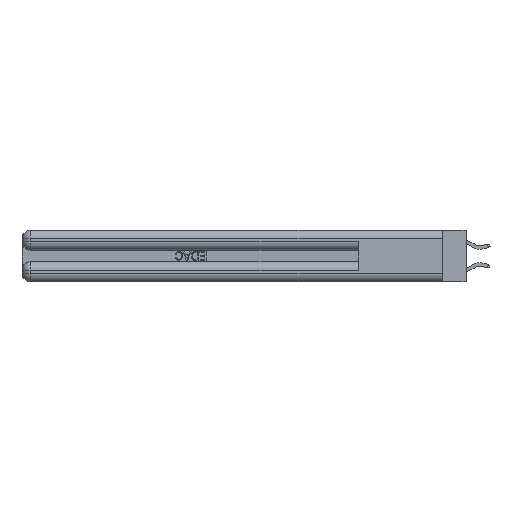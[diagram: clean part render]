
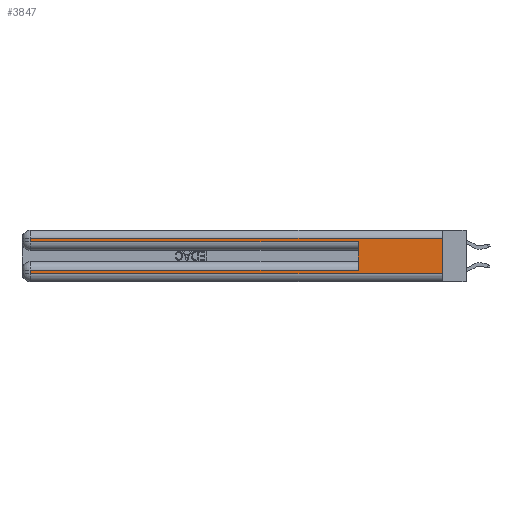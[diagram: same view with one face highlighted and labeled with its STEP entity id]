
A CAD part, left-side view. The second image highlights one B-rep face of the part: STEP entity #3847.
In plain terms, the highlighted planar face has unit normal (-1, 0, 0).
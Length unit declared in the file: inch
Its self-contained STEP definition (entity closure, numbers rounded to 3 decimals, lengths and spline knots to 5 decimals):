
#159 = VERTEX_POINT ( 'NONE', #21411 ) ;
#930 = CARTESIAN_POINT ( 'NONE',  ( 0., 2.94, 0.31 ) ) ;
#2586 = EDGE_CURVE ( 'NONE', #5223, #3981, #11230, .T. ) ;
#2915 = VECTOR ( 'NONE', #15169, 39.37008 ) ;
#3310 = DIRECTION ( 'NONE',  ( 0., 0., -1. ) ) ;
#3345 = EDGE_LOOP ( 'NONE', ( #12066, #18099, #30563, #4574, #16360, #20269, #9818, #15559 ) ) ;
#3847 = ADVANCED_FACE ( 'NONE', ( #15359 ), #16615, .F. ) ;
#3981 = VERTEX_POINT ( 'NONE', #24845 ) ;
#4574 = ORIENTED_EDGE ( 'NONE', *, *, #2586, .T. ) ;
#4626 = DIRECTION ( 'NONE',  ( 0., 0., -1. ) ) ;
#5223 = VERTEX_POINT ( 'NONE', #12116 ) ;
#5605 = EDGE_CURVE ( 'NONE', #159, #30603, #14105, .T. ) ;
#5897 = CARTESIAN_POINT ( 'NONE',  ( 0., 2.94, 0.06 ) ) ;
#6572 = EDGE_CURVE ( 'NONE', #7374, #24422, #9858, .T. ) ;
#6968 = DIRECTION ( 'NONE',  ( 1., 0., 0. ) ) ;
#7374 = VERTEX_POINT ( 'NONE', #14936 ) ;
#8783 = VERTEX_POINT ( 'NONE', #930 ) ;
#9000 = AXIS2_PLACEMENT_3D ( 'NONE', #11763, #6968, #23907 ) ;
#9295 = LINE ( 'NONE', #10842, #21410 ) ;
#9398 = LINE ( 'NONE', #12736, #2915 ) ;
#9818 = ORIENTED_EDGE ( 'NONE', *, *, #22522, .T. ) ;
#9858 = LINE ( 'NONE', #26166, #21970 ) ;
#10017 = DIRECTION ( 'NONE',  ( 0., 1., 0. ) ) ;
#10842 = CARTESIAN_POINT ( 'NONE',  ( 0., 0., 0.06 ) ) ;
#11230 = LINE ( 'NONE', #13934, #29784 ) ;
#11763 = CARTESIAN_POINT ( 'NONE',  ( 0., 0., 0.37 ) ) ;
#12066 = ORIENTED_EDGE ( 'NONE', *, *, #5605, .F. ) ;
#12116 = CARTESIAN_POINT ( 'NONE',  ( 0., 2.94, 0.285 ) ) ;
#12736 = CARTESIAN_POINT ( 'NONE',  ( 0., 0.6, 0.145 ) ) ;
#12997 = CARTESIAN_POINT ( 'NONE',  ( 0., 0., 0.37 ) ) ;
#13303 = EDGE_CURVE ( 'NONE', #8783, #5223, #31023, .T. ) ;
#13833 = DIRECTION ( 'NONE',  ( 0., -1., 0. ) ) ;
#13934 = CARTESIAN_POINT ( 'NONE',  ( 0., 0., 0.285 ) ) ;
#13986 = CARTESIAN_POINT ( 'NONE',  ( 0., 2.94, 0.085 ) ) ;
#14105 = LINE ( 'NONE', #12997, #26977 ) ;
#14798 = CARTESIAN_POINT ( 'NONE',  ( 0., 0., 0.31 ) ) ;
#14936 = CARTESIAN_POINT ( 'NONE',  ( 0., 0.6, 0.085 ) ) ;
#15169 = DIRECTION ( 'NONE',  ( 0., 0., 1. ) ) ;
#15359 = FACE_OUTER_BOUND ( 'NONE', #3345, .T. ) ;
#15382 = EDGE_CURVE ( 'NONE', #16833, #30603, #9295, .T. ) ;
#15559 = ORIENTED_EDGE ( 'NONE', *, *, #15382, .T. ) ;
#16360 = ORIENTED_EDGE ( 'NONE', *, *, #22108, .F. ) ;
#16615 = PLANE ( 'NONE',  #9000 ) ;
#16729 = CARTESIAN_POINT ( 'NONE',  ( 0., 2.94, 0.37 ) ) ;
#16833 = VERTEX_POINT ( 'NONE', #5897 ) ;
#17827 = DIRECTION ( 'NONE',  ( 0., 0., -1. ) ) ;
#18099 = ORIENTED_EDGE ( 'NONE', *, *, #23309, .T. ) ;
#18671 = CARTESIAN_POINT ( 'NONE',  ( 0., 0., 0.06 ) ) ;
#20269 = ORIENTED_EDGE ( 'NONE', *, *, #6572, .T. ) ;
#20307 = VECTOR ( 'NONE', #10017, 39.37008 ) ;
#21061 = LINE ( 'NONE', #14798, #20307 ) ;
#21408 = DIRECTION ( 'NONE',  ( 0., 1., 0. ) ) ;
#21410 = VECTOR ( 'NONE', #27868, 39.37008 ) ;
#21411 = CARTESIAN_POINT ( 'NONE',  ( 0., 0., 0.31 ) ) ;
#21970 = VECTOR ( 'NONE', #21408, 39.37008 ) ;
#22108 = EDGE_CURVE ( 'NONE', #7374, #3981, #9398, .T. ) ;
#22522 = EDGE_CURVE ( 'NONE', #24422, #16833, #23761, .T. ) ;
#23309 = EDGE_CURVE ( 'NONE', #159, #8783, #21061, .T. ) ;
#23761 = LINE ( 'NONE', #16729, #28707 ) ;
#23907 = DIRECTION ( 'NONE',  ( 0., 0., -1. ) ) ;
#24422 = VERTEX_POINT ( 'NONE', #13986 ) ;
#24554 = VECTOR ( 'NONE', #17827, 39.37008 ) ;
#24845 = CARTESIAN_POINT ( 'NONE',  ( 0., 0.6, 0.285 ) ) ;
#26166 = CARTESIAN_POINT ( 'NONE',  ( 0., 0., 0.085 ) ) ;
#26977 = VECTOR ( 'NONE', #3310, 39.37008 ) ;
#27451 = CARTESIAN_POINT ( 'NONE',  ( 0., 2.94, 0.37 ) ) ;
#27868 = DIRECTION ( 'NONE',  ( 0., -1., 0. ) ) ;
#28707 = VECTOR ( 'NONE', #4626, 39.37008 ) ;
#29784 = VECTOR ( 'NONE', #13833, 39.37008 ) ;
#30563 = ORIENTED_EDGE ( 'NONE', *, *, #13303, .T. ) ;
#30603 = VERTEX_POINT ( 'NONE', #18671 ) ;
#31023 = LINE ( 'NONE', #27451, #24554 ) ;
